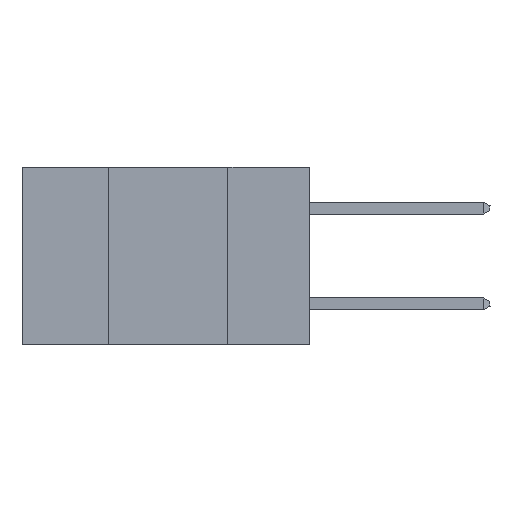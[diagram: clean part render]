
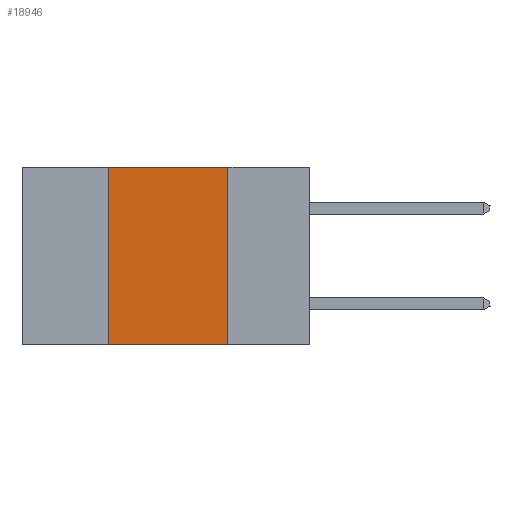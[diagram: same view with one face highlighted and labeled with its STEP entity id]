
A CAD part, left-side view. The second image highlights one B-rep face of the part: STEP entity #18946.
In plain terms, the highlighted planar face has unit normal (-1, 0, 0).
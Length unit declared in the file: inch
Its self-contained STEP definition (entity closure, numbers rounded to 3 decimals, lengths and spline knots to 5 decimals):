
#12 = VECTOR ( 'NONE', #41222, 39.37008 ) ;
#333 = ORIENTED_EDGE ( 'NONE', *, *, #10301, .F. ) ;
#759 = CARTESIAN_POINT ( 'NONE',  ( 0., 0.42, 0. ) ) ;
#1099 = DIRECTION ( 'NONE',  ( 0., 0., 1. ) ) ;
#1237 = EDGE_CURVE ( 'NONE', #32596, #27576, #11388, .T. ) ;
#2136 = AXIS2_PLACEMENT_3D ( 'NONE', #42110, #12793, #9536 ) ;
#2741 = VECTOR ( 'NONE', #8389, 39.37008 ) ;
#3481 = ORIENTED_EDGE ( 'NONE', *, *, #40811, .F. ) ;
#4058 = CARTESIAN_POINT ( 'NONE',  ( 0., 0.42, 0. ) ) ;
#7104 = LINE ( 'NONE', #12060, #12 ) ;
#7162 = CARTESIAN_POINT ( 'NONE',  ( 0., 0.6, -0.37 ) ) ;
#8389 = DIRECTION ( 'NONE',  ( 0., 0., -1. ) ) ;
#8959 = CARTESIAN_POINT ( 'NONE',  ( 0., 0.17, 0. ) ) ;
#9536 = DIRECTION ( 'NONE',  ( 0., 0., -1. ) ) ;
#10301 = EDGE_CURVE ( 'NONE', #24332, #27576, #25617, .T. ) ;
#10730 = DIRECTION ( 'NONE',  ( 0., -1., 0. ) ) ;
#11305 = EDGE_CURVE ( 'NONE', #32596, #39947, #28603, .T. ) ;
#11388 = LINE ( 'NONE', #7162, #22098 ) ;
#12060 = CARTESIAN_POINT ( 'NONE',  ( 0., 0.6, 0. ) ) ;
#12793 = DIRECTION ( 'NONE',  ( 1., 0., 0. ) ) ;
#18459 = CARTESIAN_POINT ( 'NONE',  ( 0., 0.17, -0.37 ) ) ;
#18946 = ADVANCED_FACE ( 'NONE', ( #29030 ), #19736, .F. ) ;
#19736 = PLANE ( 'NONE',  #2136 ) ;
#22098 = VECTOR ( 'NONE', #10730, 39.37008 ) ;
#24332 = VERTEX_POINT ( 'NONE', #25325 ) ;
#25325 = CARTESIAN_POINT ( 'NONE',  ( 0., 0.17, 0. ) ) ;
#25617 = LINE ( 'NONE', #8959, #2741 ) ;
#27576 = VERTEX_POINT ( 'NONE', #18459 ) ;
#28603 = LINE ( 'NONE', #4058, #38749 ) ;
#29030 = FACE_OUTER_BOUND ( 'NONE', #31292, .T. ) ;
#30859 = ORIENTED_EDGE ( 'NONE', *, *, #1237, .T. ) ;
#31292 = EDGE_LOOP ( 'NONE', ( #333, #3481, #32943, #30859 ) ) ;
#32596 = VERTEX_POINT ( 'NONE', #39083 ) ;
#32943 = ORIENTED_EDGE ( 'NONE', *, *, #11305, .F. ) ;
#38749 = VECTOR ( 'NONE', #1099, 39.37008 ) ;
#39083 = CARTESIAN_POINT ( 'NONE',  ( 0., 0.42, -0.37 ) ) ;
#39947 = VERTEX_POINT ( 'NONE', #759 ) ;
#40811 = EDGE_CURVE ( 'NONE', #39947, #24332, #7104, .T. ) ;
#41222 = DIRECTION ( 'NONE',  ( 0., -1., 0. ) ) ;
#42110 = CARTESIAN_POINT ( 'NONE',  ( 0., 0.6, 0. ) ) ;
